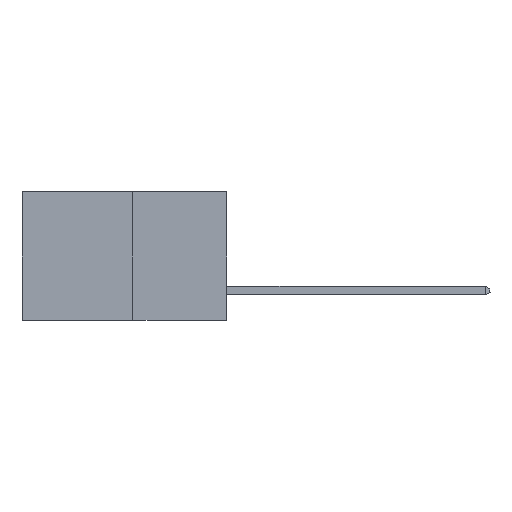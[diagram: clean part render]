
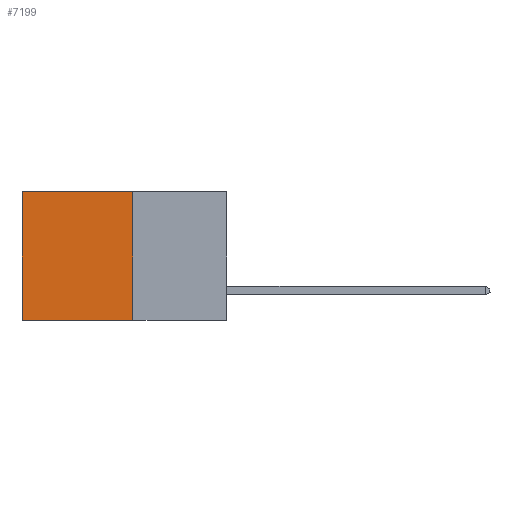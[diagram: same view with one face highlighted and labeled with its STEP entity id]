
A CAD part, left-side view. The second image highlights one B-rep face of the part: STEP entity #7199.
In plain terms, the highlighted planar face has unit normal (-1, 0, 0).
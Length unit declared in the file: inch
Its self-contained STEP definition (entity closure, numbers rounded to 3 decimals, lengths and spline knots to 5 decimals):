
#9 = CARTESIAN_POINT ( 'NONE',  ( 0.277, 0.27, 0. ) ) ;
#1283 = DIRECTION ( 'NONE',  ( 0., 0., -1. ) ) ;
#1318 = CARTESIAN_POINT ( 'NONE',  ( 0.277, 0.27, 0. ) ) ;
#2213 = ORIENTED_EDGE ( 'NONE', *, *, #16147, .F. ) ;
#2550 = LINE ( 'NONE', #9, #28587 ) ;
#3147 = VECTOR ( 'NONE', #4164, 39.37008 ) ;
#3837 = CARTESIAN_POINT ( 'NONE',  ( 0.277, 0.27, -0.37 ) ) ;
#4164 = DIRECTION ( 'NONE',  ( 0., 0., -1. ) ) ;
#4302 = AXIS2_PLACEMENT_3D ( 'NONE', #6661, #21356, #4949 ) ;
#4949 = DIRECTION ( 'NONE',  ( 0., 0., -1. ) ) ;
#6285 = VERTEX_POINT ( 'NONE', #22661 ) ;
#6451 = DIRECTION ( 'NONE',  ( 0., 1., 0. ) ) ;
#6661 = CARTESIAN_POINT ( 'NONE',  ( 0.277, 0.27, -0.37 ) ) ;
#7199 = ADVANCED_FACE ( 'NONE', ( #26051 ), #23215, .F. ) ;
#7839 = DIRECTION ( 'NONE',  ( 0., 1., 0. ) ) ;
#7962 = CARTESIAN_POINT ( 'NONE',  ( 0.277, 0.59, 0. ) ) ;
#9106 = CARTESIAN_POINT ( 'NONE',  ( 0.277, 0.27, -0.37 ) ) ;
#13762 = VERTEX_POINT ( 'NONE', #21878 ) ;
#16147 = EDGE_CURVE ( 'NONE', #27175, #13762, #17636, .T. ) ;
#17177 = EDGE_CURVE ( 'NONE', #13762, #6285, #19533, .T. ) ;
#17636 = LINE ( 'NONE', #9106, #23459 ) ;
#19117 = EDGE_CURVE ( 'NONE', #28226, #6285, #23248, .T. ) ;
#19371 = EDGE_LOOP ( 'NONE', ( #28738, #27640, #2213, #21092 ) ) ;
#19533 = LINE ( 'NONE', #3837, #25355 ) ;
#21092 = ORIENTED_EDGE ( 'NONE', *, *, #29179, .T. ) ;
#21356 = DIRECTION ( 'NONE',  ( 1., 0., 0. ) ) ;
#21796 = CARTESIAN_POINT ( 'NONE',  ( 0.277, 0.59, -0.37 ) ) ;
#21878 = CARTESIAN_POINT ( 'NONE',  ( 0.277, 0.27, -0.37 ) ) ;
#22661 = CARTESIAN_POINT ( 'NONE',  ( 0.277, 0.59, -0.37 ) ) ;
#23215 = PLANE ( 'NONE',  #4302 ) ;
#23248 = LINE ( 'NONE', #21796, #3147 ) ;
#23459 = VECTOR ( 'NONE', #1283, 39.37008 ) ;
#25355 = VECTOR ( 'NONE', #6451, 39.37008 ) ;
#26051 = FACE_OUTER_BOUND ( 'NONE', #19371, .T. ) ;
#27175 = VERTEX_POINT ( 'NONE', #1318 ) ;
#27640 = ORIENTED_EDGE ( 'NONE', *, *, #17177, .F. ) ;
#28226 = VERTEX_POINT ( 'NONE', #7962 ) ;
#28587 = VECTOR ( 'NONE', #7839, 39.37008 ) ;
#28738 = ORIENTED_EDGE ( 'NONE', *, *, #19117, .T. ) ;
#29179 = EDGE_CURVE ( 'NONE', #27175, #28226, #2550, .T. ) ;
